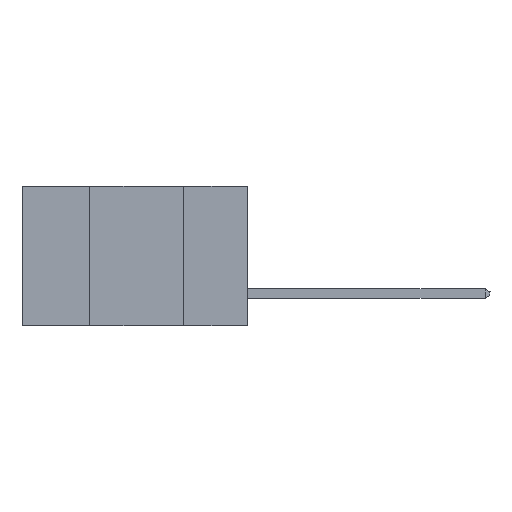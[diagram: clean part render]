
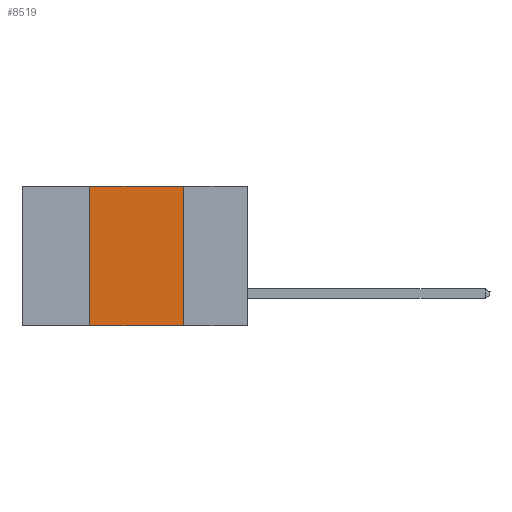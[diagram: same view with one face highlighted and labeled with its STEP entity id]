
A CAD part, left-side view. The second image highlights one B-rep face of the part: STEP entity #8519.
In plain terms, the highlighted planar face has unit normal (-1, 0, 0).
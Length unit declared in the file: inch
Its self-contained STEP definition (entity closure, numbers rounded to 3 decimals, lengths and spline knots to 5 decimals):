
#1690 = VERTEX_POINT ( 'NONE', #3086 ) ;
#2248 = ORIENTED_EDGE ( 'NONE', *, *, #3692, .F. ) ;
#2357 = AXIS2_PLACEMENT_3D ( 'NONE', #12771, #14220, #12671 ) ;
#2636 = VERTEX_POINT ( 'NONE', #15879 ) ;
#3086 = CARTESIAN_POINT ( 'NONE',  ( 0., 0.17, 0. ) ) ;
#3539 = CARTESIAN_POINT ( 'NONE',  ( 0., 0.6, 0. ) ) ;
#3692 = EDGE_CURVE ( 'NONE', #12067, #10006, #19832, .T. ) ;
#4836 = CARTESIAN_POINT ( 'NONE',  ( 0., 0.6, -0.37 ) ) ;
#4867 = FACE_OUTER_BOUND ( 'NONE', #7493, .T. ) ;
#5004 = VECTOR ( 'NONE', #9003, 39.37008 ) ;
#5082 = PLANE ( 'NONE',  #2357 ) ;
#5892 = EDGE_CURVE ( 'NONE', #12067, #2636, #8903, .T. ) ;
#6925 = LINE ( 'NONE', #19699, #7149 ) ;
#7149 = VECTOR ( 'NONE', #19594, 39.37008 ) ;
#7493 = EDGE_LOOP ( 'NONE', ( #14186, #12285, #2248, #18704 ) ) ;
#8519 = ADVANCED_FACE ( 'NONE', ( #4867 ), #5082, .F. ) ;
#8903 = LINE ( 'NONE', #4836, #5004 ) ;
#8947 = EDGE_CURVE ( 'NONE', #1690, #2636, #6925, .T. ) ;
#9003 = DIRECTION ( 'NONE',  ( 0., -1., 0. ) ) ;
#10006 = VERTEX_POINT ( 'NONE', #12178 ) ;
#11348 = LINE ( 'NONE', #3539, #12968 ) ;
#12067 = VERTEX_POINT ( 'NONE', #17061 ) ;
#12178 = CARTESIAN_POINT ( 'NONE',  ( 0., 0.42, 0. ) ) ;
#12285 = ORIENTED_EDGE ( 'NONE', *, *, #19434, .F. ) ;
#12671 = DIRECTION ( 'NONE',  ( 0., 0., -1. ) ) ;
#12771 = CARTESIAN_POINT ( 'NONE',  ( 0., 0.6, 0. ) ) ;
#12777 = DIRECTION ( 'NONE',  ( 0., -1., 0. ) ) ;
#12968 = VECTOR ( 'NONE', #12777, 39.37008 ) ;
#14186 = ORIENTED_EDGE ( 'NONE', *, *, #8947, .F. ) ;
#14220 = DIRECTION ( 'NONE',  ( 1., 0., 0. ) ) ;
#15879 = CARTESIAN_POINT ( 'NONE',  ( 0., 0.17, -0.37 ) ) ;
#16713 = CARTESIAN_POINT ( 'NONE',  ( 0., 0.42, -0.37 ) ) ;
#17018 = VECTOR ( 'NONE', #18278, 39.37008 ) ;
#17061 = CARTESIAN_POINT ( 'NONE',  ( 0., 0.42, -0.37 ) ) ;
#18278 = DIRECTION ( 'NONE',  ( 0., 0., 1. ) ) ;
#18704 = ORIENTED_EDGE ( 'NONE', *, *, #5892, .T. ) ;
#19434 = EDGE_CURVE ( 'NONE', #10006, #1690, #11348, .T. ) ;
#19594 = DIRECTION ( 'NONE',  ( 0., 0., -1. ) ) ;
#19699 = CARTESIAN_POINT ( 'NONE',  ( 0., 0.17, -0.37 ) ) ;
#19832 = LINE ( 'NONE', #16713, #17018 ) ;
